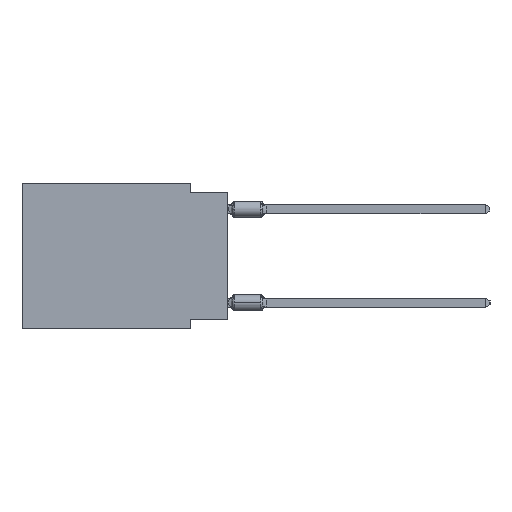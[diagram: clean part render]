
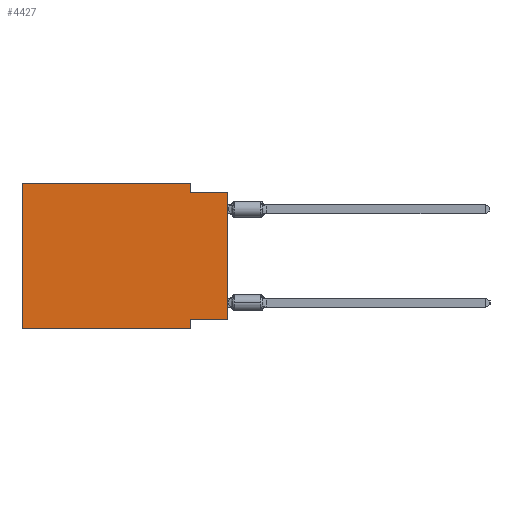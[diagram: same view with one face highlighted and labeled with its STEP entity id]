
A CAD part, left-side view. The second image highlights one B-rep face of the part: STEP entity #4427.
In plain terms, the highlighted planar face has unit normal (-1, 0, 0).
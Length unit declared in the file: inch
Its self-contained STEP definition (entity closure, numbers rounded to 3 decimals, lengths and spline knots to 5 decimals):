
#166 = LINE ( 'NONE', #10237, #28957 ) ;
#242 = LINE ( 'NONE', #23576, #30124 ) ;
#581 = VECTOR ( 'NONE', #1954, 39.37008 ) ;
#1067 = VERTEX_POINT ( 'NONE', #23764 ) ;
#1624 = ORIENTED_EDGE ( 'NONE', *, *, #15616, .F. ) ;
#1954 = DIRECTION ( 'NONE',  ( 0., -1., 0. ) ) ;
#2759 = ORIENTED_EDGE ( 'NONE', *, *, #5574, .F. ) ;
#2981 = ORIENTED_EDGE ( 'NONE', *, *, #31761, .F. ) ;
#3197 = DIRECTION ( 'NONE',  ( 0., -1., 0. ) ) ;
#4114 = LINE ( 'NONE', #13537, #29374 ) ;
#4153 = ORIENTED_EDGE ( 'NONE', *, *, #16712, .T. ) ;
#4427 = ADVANCED_FACE ( 'NONE', ( #8956 ), #18985, .F. ) ;
#4430 = CARTESIAN_POINT ( 'NONE',  ( 0., 0.55, 0. ) ) ;
#4825 = VECTOR ( 'NONE', #7998, 39.37008 ) ;
#5574 = EDGE_CURVE ( 'NONE', #14641, #31185, #21676, .T. ) ;
#5863 = CARTESIAN_POINT ( 'NONE',  ( 0., 0., -0.025 ) ) ;
#5977 = EDGE_CURVE ( 'NONE', #29438, #27183, #242, .T. ) ;
#7704 = CARTESIAN_POINT ( 'NONE',  ( 0., 0.55, -0.39 ) ) ;
#7787 = VERTEX_POINT ( 'NONE', #15668 ) ;
#7998 = DIRECTION ( 'NONE',  ( 0., 0., 1. ) ) ;
#8222 = AXIS2_PLACEMENT_3D ( 'NONE', #29514, #24559, #24245 ) ;
#8956 = FACE_OUTER_BOUND ( 'NONE', #11657, .T. ) ;
#10237 = CARTESIAN_POINT ( 'NONE',  ( 0., 0.1, -0.39 ) ) ;
#10562 = DIRECTION ( 'NONE',  ( 0., 0., -1. ) ) ;
#11657 = EDGE_LOOP ( 'NONE', ( #20802, #15640, #32484, #1624, #2759, #4153, #2981, #22192 ) ) ;
#12543 = CARTESIAN_POINT ( 'NONE',  ( 0., 0., -0.365 ) ) ;
#12723 = VECTOR ( 'NONE', #28280, 39.37008 ) ;
#13247 = LINE ( 'NONE', #13410, #17436 ) ;
#13410 = CARTESIAN_POINT ( 'NONE',  ( 0., 0.55, -0.39 ) ) ;
#13537 = CARTESIAN_POINT ( 'NONE',  ( 0., 0., -0.025 ) ) ;
#14641 = VERTEX_POINT ( 'NONE', #7704 ) ;
#15616 = EDGE_CURVE ( 'NONE', #31185, #29438, #24182, .T. ) ;
#15640 = ORIENTED_EDGE ( 'NONE', *, *, #29364, .F. ) ;
#15668 = CARTESIAN_POINT ( 'NONE',  ( 0., 0.1, -0.39 ) ) ;
#16245 = CARTESIAN_POINT ( 'NONE',  ( 0., 0.55, 0. ) ) ;
#16325 = VERTEX_POINT ( 'NONE', #5863 ) ;
#16712 = EDGE_CURVE ( 'NONE', #14641, #7787, #13247, .T. ) ;
#17063 = EDGE_CURVE ( 'NONE', #31619, #1067, #19609, .T. ) ;
#17436 = VECTOR ( 'NONE', #3197, 39.37008 ) ;
#17718 = LINE ( 'NONE', #25291, #4825 ) ;
#18240 = CARTESIAN_POINT ( 'NONE',  ( 0., 0., -0.365 ) ) ;
#18985 = PLANE ( 'NONE',  #8222 ) ;
#19609 = LINE ( 'NONE', #18240, #12723 ) ;
#20356 = CARTESIAN_POINT ( 'NONE',  ( 0., 0.1, -0.025 ) ) ;
#20802 = ORIENTED_EDGE ( 'NONE', *, *, #32527, .T. ) ;
#21676 = LINE ( 'NONE', #16245, #31712 ) ;
#22192 = ORIENTED_EDGE ( 'NONE', *, *, #17063, .F. ) ;
#23417 = DIRECTION ( 'NONE',  ( 0., 0., -1. ) ) ;
#23576 = CARTESIAN_POINT ( 'NONE',  ( 0., 0.1, 0. ) ) ;
#23655 = DIRECTION ( 'NONE',  ( 0., 0., 1. ) ) ;
#23764 = CARTESIAN_POINT ( 'NONE',  ( 0., 0.1, -0.365 ) ) ;
#24182 = LINE ( 'NONE', #4430, #581 ) ;
#24245 = DIRECTION ( 'NONE',  ( 0., 0., -1. ) ) ;
#24559 = DIRECTION ( 'NONE',  ( 1., 0., 0. ) ) ;
#25291 = CARTESIAN_POINT ( 'NONE',  ( 0., 0., 0. ) ) ;
#26184 = CARTESIAN_POINT ( 'NONE',  ( 0., 0.1, 0. ) ) ;
#26661 = DIRECTION ( 'NONE',  ( 0., -1., 0. ) ) ;
#26777 = CARTESIAN_POINT ( 'NONE',  ( 0., 0.55, 0. ) ) ;
#27183 = VERTEX_POINT ( 'NONE', #20356 ) ;
#28280 = DIRECTION ( 'NONE',  ( 0., 1., 0. ) ) ;
#28957 = VECTOR ( 'NONE', #10562, 39.37008 ) ;
#29364 = EDGE_CURVE ( 'NONE', #27183, #16325, #4114, .T. ) ;
#29374 = VECTOR ( 'NONE', #26661, 39.37008 ) ;
#29438 = VERTEX_POINT ( 'NONE', #26184 ) ;
#29514 = CARTESIAN_POINT ( 'NONE',  ( 0., 0.55, 0. ) ) ;
#30124 = VECTOR ( 'NONE', #23417, 39.37008 ) ;
#31185 = VERTEX_POINT ( 'NONE', #26777 ) ;
#31619 = VERTEX_POINT ( 'NONE', #12543 ) ;
#31712 = VECTOR ( 'NONE', #23655, 39.37008 ) ;
#31761 = EDGE_CURVE ( 'NONE', #1067, #7787, #166, .T. ) ;
#32484 = ORIENTED_EDGE ( 'NONE', *, *, #5977, .F. ) ;
#32527 = EDGE_CURVE ( 'NONE', #31619, #16325, #17718, .T. ) ;
